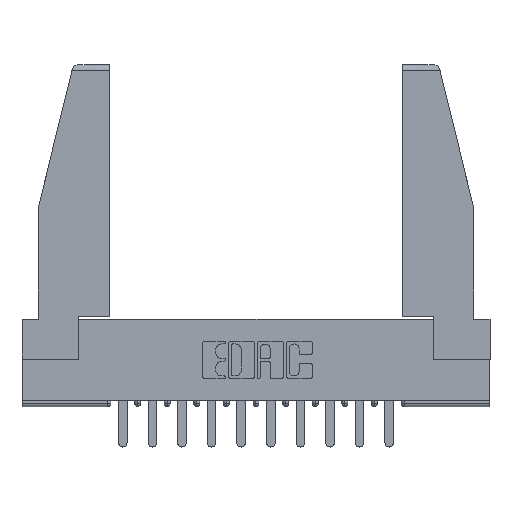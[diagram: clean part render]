
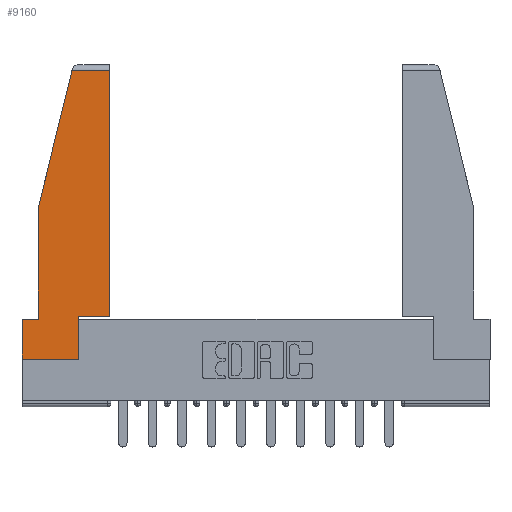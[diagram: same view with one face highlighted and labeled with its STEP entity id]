
A CAD part, top view. The second image highlights one B-rep face of the part: STEP entity #9160.
In plain terms, the highlighted planar face has unit normal (0, 0, 1).
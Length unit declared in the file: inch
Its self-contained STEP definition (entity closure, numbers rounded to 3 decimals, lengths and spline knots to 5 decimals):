
#172 = CARTESIAN_POINT ( 'NONE',  ( 0.271, 1.55, 0. ) ) ;
#697 = CARTESIAN_POINT ( 'NONE',  ( 0.086, 0.21, 0. ) ) ;
#1185 = LINE ( 'NONE', #15565, #7203 ) ;
#1199 = PLANE ( 'NONE',  #7078 ) ;
#1263 = VERTEX_POINT ( 'NONE', #11990 ) ;
#1421 = DIRECTION ( 'NONE',  ( 0., 1., 0. ) ) ;
#1684 = DIRECTION ( 'NONE',  ( -1., 0., 0. ) ) ;
#1893 = VECTOR ( 'NONE', #15518, 39.37008 ) ;
#1912 = VERTEX_POINT ( 'NONE', #697 ) ;
#2052 = LINE ( 'NONE', #172, #9733 ) ;
#2256 = EDGE_CURVE ( 'NONE', #14061, #3301, #6402, .T. ) ;
#2279 = LINE ( 'NONE', #9227, #10579 ) ;
#2325 = VERTEX_POINT ( 'NONE', #3368 ) ;
#2405 = CARTESIAN_POINT ( 'NONE',  ( 0., 0., 0. ) ) ;
#2571 = CARTESIAN_POINT ( 'NONE',  ( 0.461, 0.223, 0. ) ) ;
#3210 = CARTESIAN_POINT ( 'NONE',  ( 0.2636, 1.52, 0. ) ) ;
#3301 = VERTEX_POINT ( 'NONE', #3210 ) ;
#3368 = CARTESIAN_POINT ( 'NONE',  ( 0.297, 0., 0. ) ) ;
#3678 = LINE ( 'NONE', #4360, #12968 ) ;
#3919 = VERTEX_POINT ( 'NONE', #13825 ) ;
#3967 = CARTESIAN_POINT ( 'NONE',  ( 0.297, 0., 0. ) ) ;
#3986 = DIRECTION ( 'NONE',  ( 1., 0., 0. ) ) ;
#4360 = CARTESIAN_POINT ( 'NONE',  ( 0., 0.21, 0. ) ) ;
#4993 = VECTOR ( 'NONE', #11300, 39.37008 ) ;
#5041 = FACE_OUTER_BOUND ( 'NONE', #10820, .T. ) ;
#5221 = EDGE_CURVE ( 'NONE', #1263, #12805, #16730, .T. ) ;
#5333 = EDGE_CURVE ( 'NONE', #12805, #14061, #2279, .T. ) ;
#5919 = LINE ( 'NONE', #3967, #11919 ) ;
#6099 = CARTESIAN_POINT ( 'NONE',  ( 0.297, 0.223, 0. ) ) ;
#6402 = LINE ( 'NONE', #11346, #10150 ) ;
#6654 = CARTESIAN_POINT ( 'NONE',  ( 0., 0.21, 0. ) ) ;
#7078 = AXIS2_PLACEMENT_3D ( 'NONE', #13218, #10466, #3986 ) ;
#7203 = VECTOR ( 'NONE', #10212, 39.37008 ) ;
#7784 = DIRECTION ( 'NONE',  ( -1., 0., 0. ) ) ;
#7846 = ORIENTED_EDGE ( 'NONE', *, *, #14247, .T. ) ;
#7954 = ORIENTED_EDGE ( 'NONE', *, *, #5221, .T. ) ;
#8693 = EDGE_CURVE ( 'NONE', #2325, #1263, #5919, .T. ) ;
#8962 = CARTESIAN_POINT ( 'NONE',  ( 0., 0.21, 0. ) ) ;
#9152 = LINE ( 'NONE', #8962, #1893 ) ;
#9160 = ADVANCED_FACE ( 'NONE', ( #5041 ), #1199, .T. ) ;
#9227 = CARTESIAN_POINT ( 'NONE',  ( 0.461, 0.223, 0. ) ) ;
#9370 = DIRECTION ( 'NONE',  ( -0.239, -0.971, 0. ) ) ;
#9733 = VECTOR ( 'NONE', #9370, 39.37008 ) ;
#10150 = VECTOR ( 'NONE', #7784, 39.37008 ) ;
#10212 = DIRECTION ( 'NONE',  ( 0., -1., 0. ) ) ;
#10466 = DIRECTION ( 'NONE',  ( 0., 0., 1. ) ) ;
#10579 = VECTOR ( 'NONE', #11987, 39.37008 ) ;
#10820 = EDGE_LOOP ( 'NONE', ( #14329, #14434, #7846, #12724, #15311, #12176, #15959, #11471, #7954 ) ) ;
#10938 = VECTOR ( 'NONE', #16071, 39.37008 ) ;
#11300 = DIRECTION ( 'NONE',  ( 1., 0., 0. ) ) ;
#11346 = CARTESIAN_POINT ( 'NONE',  ( 0., 1.52, 0. ) ) ;
#11471 = ORIENTED_EDGE ( 'NONE', *, *, #8693, .T. ) ;
#11798 = CARTESIAN_POINT ( 'NONE',  ( 0., 0., 0. ) ) ;
#11919 = VECTOR ( 'NONE', #1421, 39.37008 ) ;
#11959 = LINE ( 'NONE', #11798, #10938 ) ;
#11987 = DIRECTION ( 'NONE',  ( 0., 1., 0. ) ) ;
#11990 = CARTESIAN_POINT ( 'NONE',  ( 0.297, 0.223, 0. ) ) ;
#12176 = ORIENTED_EDGE ( 'NONE', *, *, #13147, .T. ) ;
#12261 = CARTESIAN_POINT ( 'NONE',  ( 0.461, 1.52, 0. ) ) ;
#12724 = ORIENTED_EDGE ( 'NONE', *, *, #16974, .T. ) ;
#12725 = VERTEX_POINT ( 'NONE', #2405 ) ;
#12805 = VERTEX_POINT ( 'NONE', #2571 ) ;
#12968 = VECTOR ( 'NONE', #1684, 39.37008 ) ;
#13147 = EDGE_CURVE ( 'NONE', #13893, #12725, #9152, .T. ) ;
#13218 = CARTESIAN_POINT ( 'NONE',  ( 0., 0., 0. ) ) ;
#13825 = CARTESIAN_POINT ( 'NONE',  ( 0.086, 0.8, 0. ) ) ;
#13893 = VERTEX_POINT ( 'NONE', #6654 ) ;
#14061 = VERTEX_POINT ( 'NONE', #12261 ) ;
#14247 = EDGE_CURVE ( 'NONE', #3301, #3919, #2052, .T. ) ;
#14329 = ORIENTED_EDGE ( 'NONE', *, *, #5333, .T. ) ;
#14434 = ORIENTED_EDGE ( 'NONE', *, *, #2256, .T. ) ;
#15140 = EDGE_CURVE ( 'NONE', #12725, #2325, #11959, .T. ) ;
#15231 = EDGE_CURVE ( 'NONE', #1912, #13893, #3678, .T. ) ;
#15311 = ORIENTED_EDGE ( 'NONE', *, *, #15231, .T. ) ;
#15518 = DIRECTION ( 'NONE',  ( 0., -1., 0. ) ) ;
#15565 = CARTESIAN_POINT ( 'NONE',  ( 0.086, 0.8, 0. ) ) ;
#15959 = ORIENTED_EDGE ( 'NONE', *, *, #15140, .T. ) ;
#16071 = DIRECTION ( 'NONE',  ( 1., 0., 0. ) ) ;
#16730 = LINE ( 'NONE', #6099, #4993 ) ;
#16974 = EDGE_CURVE ( 'NONE', #3919, #1912, #1185, .T. ) ;
